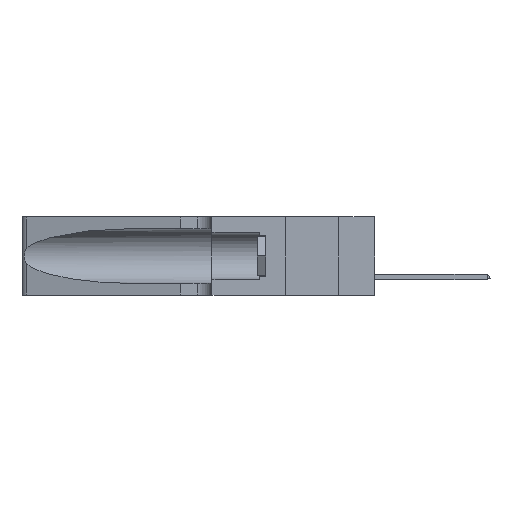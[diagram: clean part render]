
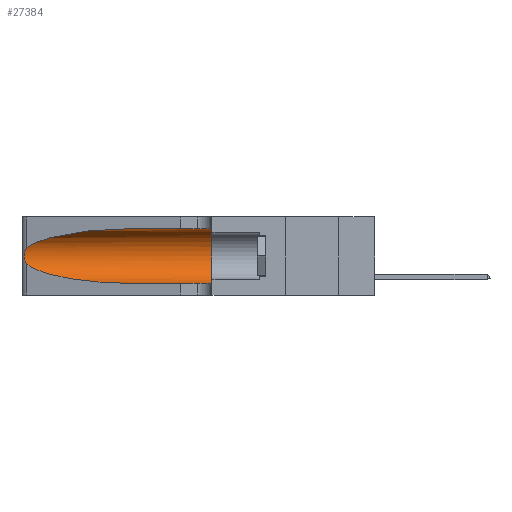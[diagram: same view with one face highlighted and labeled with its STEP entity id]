
A CAD part, left-side view. The second image highlights one B-rep face of the part: STEP entity #27384.
In plain terms, the highlighted cylindrical face has radius 3.308 mm (diameter 6.617 mm), a partial arc.
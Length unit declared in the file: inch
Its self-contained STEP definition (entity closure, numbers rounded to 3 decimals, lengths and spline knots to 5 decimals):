
#1534 = CARTESIAN_POINT ( 'NONE',  ( 0.26075, 1.23896, 0.19203 ) ) ;
#1701 = CARTESIAN_POINT ( 'NONE',  ( 0.26017, 1.23833, 0.17102 ) ) ;
#1720 = ORIENTED_EDGE ( 'NONE', *, *, #23278, .T. ) ;
#2768 = EDGE_CURVE ( 'NONE', #26275, #3174, #8042, .T. ) ;
#3174 = VERTEX_POINT ( 'NONE', #34470 ) ;
#3455 = DIRECTION ( 'NONE',  ( 0., 0., -1. ) ) ;
#3763 = CARTESIAN_POINT ( 'NONE',  ( 0.1305, 1.61858, 0.31525 ) ) ;
#3890 = FACE_OUTER_BOUND ( 'NONE', #33419, .T. ) ;
#4573 = CARTESIAN_POINT ( 'NONE',  ( 0.2373, 1.15595, 0.28018 ) ) ;
#5245 = CARTESIAN_POINT ( 'NONE',  ( 0.26075, 1.23896, 0.178 ) ) ;
#6537 = EDGE_CURVE ( 'NONE', #37931, #3174, #38006, .T. ) ;
#6703 = CARTESIAN_POINT ( 'NONE',  ( 0.1305, 0.35, 0.31525 ) ) ;
#7288 = AXIS2_PLACEMENT_3D ( 'NONE', #17108, #25539, #3455 ) ;
#8042 = LINE ( 'NONE', #24755, #9203 ) ;
#8299 = ORIENTED_EDGE ( 'NONE', *, *, #2768, .T. ) ;
#8467 = CARTESIAN_POINT ( 'NONE',  ( 0.25487, 1.22718, 0.22369 ) ) ;
#8959 = CARTESIAN_POINT ( 'NONE',  ( 0.25487, 1.22718, 0.14631 ) ) ;
#9044 = VERTEX_POINT ( 'NONE', #27421 ) ;
#9203 = VECTOR ( 'NONE', #13903, 39.37008 ) ;
#12159 = CARTESIAN_POINT ( 'NONE',  ( 0.25555, 1.22994, 0.2215 ) ) ;
#12450 = B_SPLINE_CURVE_WITH_KNOTS ( 'NONE', 3,
 ( #8467, #12159, #19988, #45294, #16466, #23666, #1534, #5245, #1701, #23340, #42101, #45786, #30854, #8959 ),
 .UNSPECIFIED., .F., .F.,
 ( 4, 2, 2, 2, 2, 2, 4 ),
 ( 0., 0.00027, 0.00053, 0.00107, 0.0016, 0.00187, 0.00214 ),
 .UNSPECIFIED. ) ;
#13126 = CYLINDRICAL_SURFACE ( 'NONE', #7288, 0.13025 ) ;
#13215 = CARTESIAN_POINT ( 'NONE',  ( 0.25487, 1.22718, 0.14631 ) ) ;
#13903 = DIRECTION ( 'NONE',  ( 0., -1., 0. ) ) ;
#16466 = CARTESIAN_POINT ( 'NONE',  ( 0.25854, 1.2359, 0.20912 ) ) ;
#17108 = CARTESIAN_POINT ( 'NONE',  ( 0.1305, 1.61858, 0.185 ) ) ;
#17378 = VECTOR ( 'NONE', #47345, 39.37008 ) ;
#19325 = CARTESIAN_POINT ( 'NONE',  ( 0.1305, 0.72297, 0.31525 ) ) ;
#19670 = CARTESIAN_POINT ( 'NONE',  ( 0.18966, 0.96281, 0.05475 ) ) ;
#19988 = CARTESIAN_POINT ( 'NONE',  ( 0.25639, 1.23184, 0.21858 ) ) ;
#20365 = ORIENTED_EDGE ( 'NONE', *, *, #42522, .F. ) ;
#21826 = EDGE_CURVE ( 'NONE', #42887, #26275, #37372, .T. ) ;
#22835 = CARTESIAN_POINT ( 'NONE',  ( 0.18966, 0.96281, 0.31525 ) ) ;
#23020 = CARTESIAN_POINT ( 'NONE',  ( 0.1305, 0.72297, 0.05475 ) ) ;
#23163 = DIRECTION ( 'NONE',  ( 0., 1., 0. ) ) ;
#23278 = EDGE_CURVE ( 'NONE', #47436, #42887, #12450, .T. ) ;
#23340 = CARTESIAN_POINT ( 'NONE',  ( 0.25856, 1.23593, 0.16098 ) ) ;
#23666 = CARTESIAN_POINT ( 'NONE',  ( 0.26018, 1.23835, 0.19895 ) ) ;
#24520 = ORIENTED_EDGE ( 'NONE', *, *, #6537, .F. ) ;
#24755 = CARTESIAN_POINT ( 'NONE',  ( 0.1305, 1.61858, 0.05475 ) ) ;
#24955 = ORIENTED_EDGE ( 'NONE', *, *, #21826, .T. ) ;
#25539 = DIRECTION ( 'NONE',  ( 0., -1., 0. ) ) ;
#26225 = CARTESIAN_POINT ( 'NONE',  ( 0.1305, 0.72297, 0.05475 ) ) ;
#26275 = VERTEX_POINT ( 'NONE', #26225 ) ;
#26807 = DIRECTION ( 'NONE',  ( 0., 0., 1. ) ) ;
#26975 = CARTESIAN_POINT ( 'NONE',  ( 0.2373, 1.15595, 0.08982 ) ) ;
#27384 = ADVANCED_FACE ( 'NONE', ( #3890 ), #13126, .F. ) ;
#27421 = CARTESIAN_POINT ( 'NONE',  ( 0.1305, 0.72297, 0.31525 ) ) ;
#28794 =( BOUNDED_CURVE ( )  B_SPLINE_CURVE ( 3, ( #19325, #22835, #4573, #37581 ),
 .UNSPECIFIED., .F., .F. ) 
 B_SPLINE_CURVE_WITH_KNOTS ( ( 4, 4 ),
 ( 1.5708, 2.84003 ),
 .UNSPECIFIED. ) 
 CURVE ( )  GEOMETRIC_REPRESENTATION_ITEM ( )  RATIONAL_B_SPLINE_CURVE ( ( 1., 0.87, 0.87, 1. ) ) 
 REPRESENTATION_ITEM ( '' )  );
#29164 = ORIENTED_EDGE ( 'NONE', *, *, #30360, .T. ) ;
#30360 = EDGE_CURVE ( 'NONE', #9044, #47436, #28794, .T. ) ;
#30854 = CARTESIAN_POINT ( 'NONE',  ( 0.25555, 1.22993, 0.14849 ) ) ;
#33419 = EDGE_LOOP ( 'NONE', ( #29164, #1720, #24955, #8299, #24520, #20365 ) ) ;
#34175 = AXIS2_PLACEMENT_3D ( 'NONE', #45783, #23163, #26807 ) ;
#34470 = CARTESIAN_POINT ( 'NONE',  ( 0.1305, 0.35, 0.05475 ) ) ;
#34507 = CARTESIAN_POINT ( 'NONE',  ( 0.25487, 1.22718, 0.22369 ) ) ;
#37372 =( BOUNDED_CURVE ( )  B_SPLINE_CURVE ( 3, ( #44979, #26975, #19670, #23020 ),
 .UNSPECIFIED., .F., .T. ) 
 B_SPLINE_CURVE_WITH_KNOTS ( ( 4, 4 ),
 ( 3.44316, 4.71239 ),
 .UNSPECIFIED. ) 
 CURVE ( )  GEOMETRIC_REPRESENTATION_ITEM ( )  RATIONAL_B_SPLINE_CURVE ( ( 1., 0.87, 0.87, 1. ) ) 
 REPRESENTATION_ITEM ( '' )  );
#37581 = CARTESIAN_POINT ( 'NONE',  ( 0.25487, 1.22718, 0.22369 ) ) ;
#37931 = VERTEX_POINT ( 'NONE', #6703 ) ;
#38006 = CIRCLE ( 'NONE', #34175, 0.13025 ) ;
#40302 = LINE ( 'NONE', #3763, #17378 ) ;
#42101 = CARTESIAN_POINT ( 'NONE',  ( 0.25789, 1.23486, 0.15765 ) ) ;
#42522 = EDGE_CURVE ( 'NONE', #9044, #37931, #40302, .T. ) ;
#42887 = VERTEX_POINT ( 'NONE', #13215 ) ;
#44979 = CARTESIAN_POINT ( 'NONE',  ( 0.25487, 1.22718, 0.14631 ) ) ;
#45294 = CARTESIAN_POINT ( 'NONE',  ( 0.25787, 1.23484, 0.2124 ) ) ;
#45783 = CARTESIAN_POINT ( 'NONE',  ( 0.1305, 0.35, 0.185 ) ) ;
#45786 = CARTESIAN_POINT ( 'NONE',  ( 0.25639, 1.23186, 0.15144 ) ) ;
#47345 = DIRECTION ( 'NONE',  ( 0., -1., 0. ) ) ;
#47436 = VERTEX_POINT ( 'NONE', #34507 ) ;
